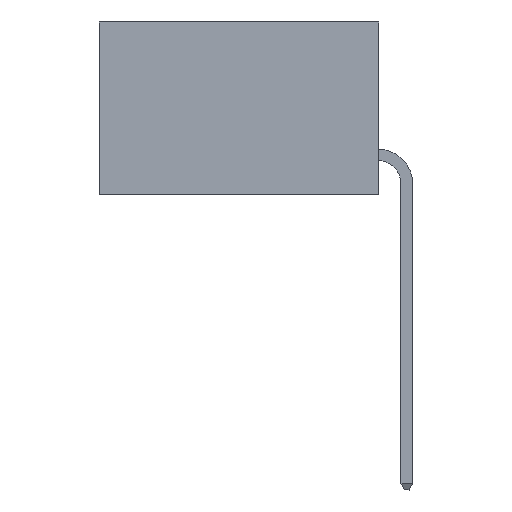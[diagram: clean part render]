
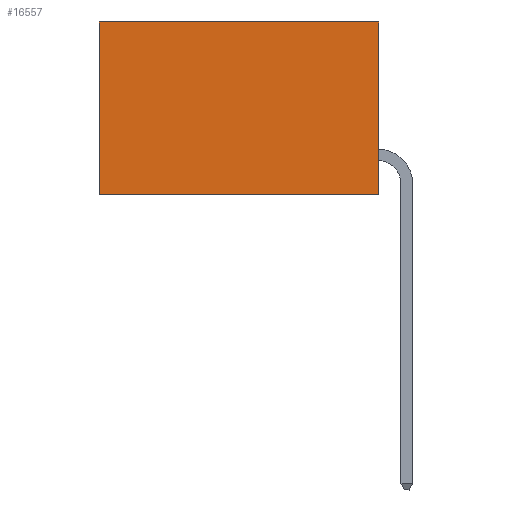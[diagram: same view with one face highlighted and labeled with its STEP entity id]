
A CAD part, left-side view. The second image highlights one B-rep face of the part: STEP entity #16557.
In plain terms, the highlighted planar face has unit normal (-1, 0, 0).
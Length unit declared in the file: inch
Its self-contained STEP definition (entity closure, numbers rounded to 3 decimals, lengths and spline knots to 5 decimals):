
#178 = DIRECTION ( 'NONE',  ( 0., 1., 0. ) ) ;
#528 = VECTOR ( 'NONE', #1285, 39.37008 ) ;
#1087 = ORIENTED_EDGE ( 'NONE', *, *, #2274, .F. ) ;
#1285 = DIRECTION ( 'NONE',  ( 0., 0., -1. ) ) ;
#2274 = EDGE_CURVE ( 'NONE', #2472, #7953, #8846, .T. ) ;
#2472 = VERTEX_POINT ( 'NONE', #13654 ) ;
#2653 = DIRECTION ( 'NONE',  ( 0., 0., -1. ) ) ;
#2934 = CARTESIAN_POINT ( 'NONE',  ( 0.2615, 0., -0.37 ) ) ;
#3381 = ORIENTED_EDGE ( 'NONE', *, *, #5761, .T. ) ;
#3709 = FACE_OUTER_BOUND ( 'NONE', #14645, .T. ) ;
#4614 = CARTESIAN_POINT ( 'NONE',  ( 0.2615, 0., -0.37 ) ) ;
#5092 = DIRECTION ( 'NONE',  ( 0., 0., -1. ) ) ;
#5112 = CARTESIAN_POINT ( 'NONE',  ( 0.2615, 0.6, -0.37 ) ) ;
#5430 = CARTESIAN_POINT ( 'NONE',  ( 0.2615, 0., 0. ) ) ;
#5654 = AXIS2_PLACEMENT_3D ( 'NONE', #6456, #17754, #5092 ) ;
#5761 = EDGE_CURVE ( 'NONE', #12259, #7953, #9490, .T. ) ;
#6227 = ORIENTED_EDGE ( 'NONE', *, *, #10007, .F. ) ;
#6456 = CARTESIAN_POINT ( 'NONE',  ( 0.2615, 0., -0.37 ) ) ;
#7201 = EDGE_CURVE ( 'NONE', #11882, #12259, #17334, .T. ) ;
#7359 = DIRECTION ( 'NONE',  ( 0., 1., 0. ) ) ;
#7953 = VERTEX_POINT ( 'NONE', #5112 ) ;
#8846 = LINE ( 'NONE', #4614, #14204 ) ;
#8992 = VECTOR ( 'NONE', #2653, 39.37008 ) ;
#9231 = PLANE ( 'NONE',  #5654 ) ;
#9490 = LINE ( 'NONE', #15126, #528 ) ;
#10007 = EDGE_CURVE ( 'NONE', #11882, #2472, #15292, .T. ) ;
#10488 = CARTESIAN_POINT ( 'NONE',  ( 0.2615, 0.6, 0. ) ) ;
#11787 = ORIENTED_EDGE ( 'NONE', *, *, #7201, .T. ) ;
#11882 = VERTEX_POINT ( 'NONE', #5430 ) ;
#12259 = VERTEX_POINT ( 'NONE', #10488 ) ;
#13654 = CARTESIAN_POINT ( 'NONE',  ( 0.2615, 0., -0.37 ) ) ;
#14204 = VECTOR ( 'NONE', #7359, 39.37008 ) ;
#14217 = CARTESIAN_POINT ( 'NONE',  ( 0.2615, 0., 0. ) ) ;
#14645 = EDGE_LOOP ( 'NONE', ( #3381, #1087, #6227, #11787 ) ) ;
#15126 = CARTESIAN_POINT ( 'NONE',  ( 0.2615, 0.6, -0.37 ) ) ;
#15292 = LINE ( 'NONE', #2934, #8992 ) ;
#16557 = ADVANCED_FACE ( 'NONE', ( #3709 ), #9231, .F. ) ;
#17334 = LINE ( 'NONE', #14217, #17882 ) ;
#17754 = DIRECTION ( 'NONE',  ( 1., 0., 0. ) ) ;
#17882 = VECTOR ( 'NONE', #178, 39.37008 ) ;
